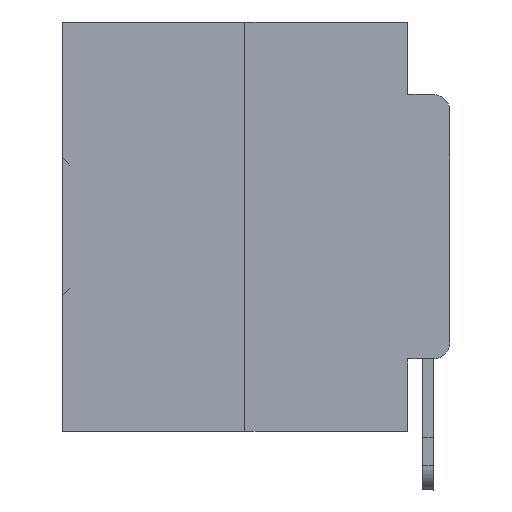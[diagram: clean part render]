
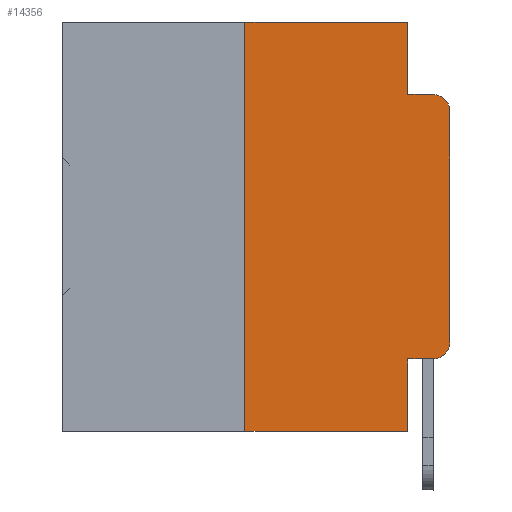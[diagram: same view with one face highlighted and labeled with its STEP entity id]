
A CAD part, left-side view. The second image highlights one B-rep face of the part: STEP entity #14356.
In plain terms, the highlighted planar face has unit normal (-1, 0, 0).
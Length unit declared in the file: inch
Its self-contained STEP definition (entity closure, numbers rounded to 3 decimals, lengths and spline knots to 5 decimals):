
#647 = VECTOR ( 'NONE', #10222, 39.37008 ) ;
#802 = DIRECTION ( 'NONE',  ( 0., 0., -1. ) ) ;
#943 = VERTEX_POINT ( 'NONE', #25394 ) ;
#1159 = EDGE_CURVE ( 'NONE', #9414, #7683, #20958, .T. ) ;
#1272 = CARTESIAN_POINT ( 'NONE',  ( 0., 0.473, 0. ) ) ;
#1504 = LINE ( 'NONE', #9861, #647 ) ;
#2055 = ORIENTED_EDGE ( 'NONE', *, *, #15174, .T. ) ;
#2188 = DIRECTION ( 'NONE',  ( 0., 0., -1. ) ) ;
#3841 = EDGE_CURVE ( 'NONE', #25967, #18893, #7540, .T. ) ;
#4926 = DIRECTION ( 'NONE',  ( 0., -1., 0. ) ) ;
#5937 = ORIENTED_EDGE ( 'NONE', *, *, #7384, .T. ) ;
#5998 = LINE ( 'NONE', #17327, #32028 ) ;
#6430 = ORIENTED_EDGE ( 'NONE', *, *, #3841, .T. ) ;
#6494 = EDGE_LOOP ( 'NONE', ( #26249, #5937, #18872, #32822, #29227, #24209, #6430, #22317, #29424, #2055 ) ) ;
#6629 = CARTESIAN_POINT ( 'NONE',  ( 0., 0.051, 0. ) ) ;
#7384 = EDGE_CURVE ( 'NONE', #16796, #10884, #13369, .T. ) ;
#7540 = LINE ( 'NONE', #7909, #30511 ) ;
#7683 = VERTEX_POINT ( 'NONE', #6629 ) ;
#7909 = CARTESIAN_POINT ( 'NONE',  ( 0., 0.473, -0.5 ) ) ;
#8047 = AXIS2_PLACEMENT_3D ( 'NONE', #25006, #35755, #2188 ) ;
#8353 = CARTESIAN_POINT ( 'NONE',  ( 0., 0.051, -0.5 ) ) ;
#9410 = CARTESIAN_POINT ( 'NONE',  ( 0., 0.02, -0.0885 ) ) ;
#9414 = VERTEX_POINT ( 'NONE', #25348 ) ;
#9524 = VERTEX_POINT ( 'NONE', #16836 ) ;
#9861 = CARTESIAN_POINT ( 'NONE',  ( 0., 0.051, 0. ) ) ;
#10222 = DIRECTION ( 'NONE',  ( 0., 0., -1. ) ) ;
#10649 = EDGE_CURVE ( 'NONE', #9524, #10884, #30736, .T. ) ;
#10810 = FACE_OUTER_BOUND ( 'NONE', #6494, .T. ) ;
#10884 = VERTEX_POINT ( 'NONE', #9410 ) ;
#12970 = AXIS2_PLACEMENT_3D ( 'NONE', #14720, #26209, #802 ) ;
#13369 = CIRCLE ( 'NONE', #8047, 0.02 ) ;
#13402 = VECTOR ( 'NONE', #29391, 39.37008 ) ;
#14146 = AXIS2_PLACEMENT_3D ( 'NONE', #24530, #16376, #33060 ) ;
#14356 = ADVANCED_FACE ( 'NONE', ( #10810 ), #25262, .F. ) ;
#14720 = CARTESIAN_POINT ( 'NONE',  ( 0., 0.02, -0.3915 ) ) ;
#15174 = EDGE_CURVE ( 'NONE', #34963, #16046, #18317, .T. ) ;
#15444 = EDGE_CURVE ( 'NONE', #943, #34963, #30812, .T. ) ;
#15685 = CARTESIAN_POINT ( 'NONE',  ( 0., 0., -0.1085 ) ) ;
#15902 = EDGE_CURVE ( 'NONE', #7683, #9524, #22084, .T. ) ;
#16046 = VERTEX_POINT ( 'NONE', #36514 ) ;
#16376 = DIRECTION ( 'NONE',  ( 1., 0., 0. ) ) ;
#16796 = VERTEX_POINT ( 'NONE', #15685 ) ;
#16836 = CARTESIAN_POINT ( 'NONE',  ( 0., 0.051, -0.0885 ) ) ;
#16902 = EDGE_CURVE ( 'NONE', #16046, #16796, #5998, .T. ) ;
#17327 = CARTESIAN_POINT ( 'NONE',  ( 0., 0., 0. ) ) ;
#18115 = CARTESIAN_POINT ( 'NONE',  ( 0., 0.25, 0. ) ) ;
#18317 = CIRCLE ( 'NONE', #12970, 0.02 ) ;
#18748 = EDGE_CURVE ( 'NONE', #943, #18893, #1504, .T. ) ;
#18872 = ORIENTED_EDGE ( 'NONE', *, *, #10649, .F. ) ;
#18893 = VERTEX_POINT ( 'NONE', #8353 ) ;
#19076 = CARTESIAN_POINT ( 'NONE',  ( 0., 0.051, -0.0885 ) ) ;
#19768 = DIRECTION ( 'NONE',  ( 0., 0., 1. ) ) ;
#20958 = LINE ( 'NONE', #1272, #32245 ) ;
#21528 = DIRECTION ( 'NONE',  ( 0., 0., -1. ) ) ;
#21574 = VECTOR ( 'NONE', #36483, 39.37008 ) ;
#22084 = LINE ( 'NONE', #24293, #28999 ) ;
#22317 = ORIENTED_EDGE ( 'NONE', *, *, #18748, .F. ) ;
#22985 = DIRECTION ( 'NONE',  ( 0., -1., 0. ) ) ;
#23670 = LINE ( 'NONE', #18115, #13402 ) ;
#24209 = ORIENTED_EDGE ( 'NONE', *, *, #33565, .F. ) ;
#24242 = VECTOR ( 'NONE', #24701, 39.37008 ) ;
#24293 = CARTESIAN_POINT ( 'NONE',  ( 0., 0.051, 0. ) ) ;
#24530 = CARTESIAN_POINT ( 'NONE',  ( 0., 0.473, 0. ) ) ;
#24701 = DIRECTION ( 'NONE',  ( 0., -1., 0. ) ) ;
#25006 = CARTESIAN_POINT ( 'NONE',  ( 0., 0.02, -0.1085 ) ) ;
#25262 = PLANE ( 'NONE',  #14146 ) ;
#25348 = CARTESIAN_POINT ( 'NONE',  ( 0., 0.25, 0. ) ) ;
#25394 = CARTESIAN_POINT ( 'NONE',  ( 0., 0.051, -0.4115 ) ) ;
#25967 = VERTEX_POINT ( 'NONE', #26553 ) ;
#26209 = DIRECTION ( 'NONE',  ( -1., 0., 0. ) ) ;
#26249 = ORIENTED_EDGE ( 'NONE', *, *, #16902, .T. ) ;
#26553 = CARTESIAN_POINT ( 'NONE',  ( 0., 0.25, -0.5 ) ) ;
#28025 = CARTESIAN_POINT ( 'NONE',  ( 0., 0.051, -0.4115 ) ) ;
#28999 = VECTOR ( 'NONE', #21528, 39.37008 ) ;
#29227 = ORIENTED_EDGE ( 'NONE', *, *, #1159, .F. ) ;
#29391 = DIRECTION ( 'NONE',  ( 0., 0., 1. ) ) ;
#29424 = ORIENTED_EDGE ( 'NONE', *, *, #15444, .T. ) ;
#30511 = VECTOR ( 'NONE', #4926, 39.37008 ) ;
#30736 = LINE ( 'NONE', #19076, #21574 ) ;
#30812 = LINE ( 'NONE', #28025, #24242 ) ;
#32028 = VECTOR ( 'NONE', #19768, 39.37008 ) ;
#32245 = VECTOR ( 'NONE', #22985, 39.37008 ) ;
#32822 = ORIENTED_EDGE ( 'NONE', *, *, #15902, .F. ) ;
#33060 = DIRECTION ( 'NONE',  ( 0., 0., -1. ) ) ;
#33320 = CARTESIAN_POINT ( 'NONE',  ( 0., 0.02, -0.4115 ) ) ;
#33565 = EDGE_CURVE ( 'NONE', #25967, #9414, #23670, .T. ) ;
#34963 = VERTEX_POINT ( 'NONE', #33320 ) ;
#35755 = DIRECTION ( 'NONE',  ( -1., 0., 0. ) ) ;
#36483 = DIRECTION ( 'NONE',  ( 0., -1., 0. ) ) ;
#36514 = CARTESIAN_POINT ( 'NONE',  ( 0., 0., -0.3915 ) ) ;
